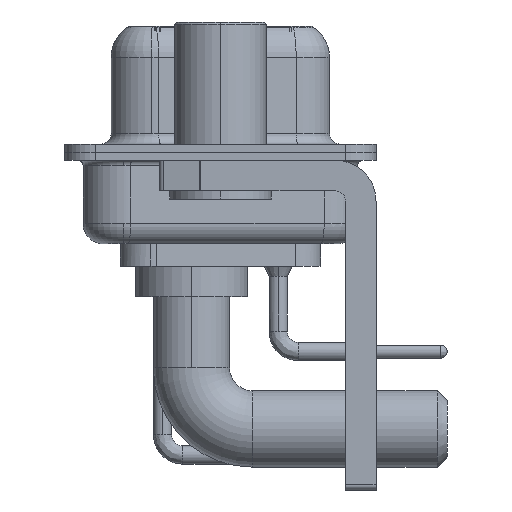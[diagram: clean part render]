
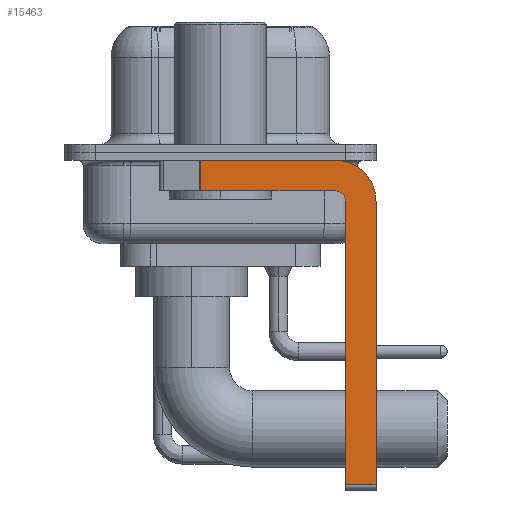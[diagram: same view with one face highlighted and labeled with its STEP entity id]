
A CAD part, left-side view. The second image highlights one B-rep face of the part: STEP entity #15463.
In plain terms, the highlighted planar face has unit normal (-1, 0, 0).
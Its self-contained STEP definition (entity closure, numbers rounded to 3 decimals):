
#171 = EDGE_LOOP ( 'NONE', ( #15192, #24403, #6575, #6069, #23442, #17105, #9714, #32960 ) ) ;
#210 = EDGE_CURVE ( 'NONE', #28596, #7166, #14443, .T. ) ;
#306 = LINE ( 'NONE', #27410, #15959 ) ;
#643 = DIRECTION ( 'NONE',  ( 0., 0., -1. ) ) ;
#693 = LINE ( 'NONE', #11523, #34291 ) ;
#996 = VERTEX_POINT ( 'NONE', #18488 ) ;
#1873 = DIRECTION ( 'NONE',  ( -1., 0., 0. ) ) ;
#3030 = VERTEX_POINT ( 'NONE', #29535 ) ;
#4671 = AXIS2_PLACEMENT_3D ( 'NONE', #13766, #25094, #643 ) ;
#4718 = DIRECTION ( 'NONE',  ( 0., 1., 0. ) ) ;
#5029 = FACE_OUTER_BOUND ( 'NONE', #171, .T. ) ;
#5260 = CARTESIAN_POINT ( 'NONE',  ( -2.9, -5.65, -0.4 ) ) ;
#6069 = ORIENTED_EDGE ( 'NONE', *, *, #210, .F. ) ;
#6180 = CARTESIAN_POINT ( 'NONE',  ( -2.9, -6.15, -2.4 ) ) ;
#6575 = ORIENTED_EDGE ( 'NONE', *, *, #10135, .F. ) ;
#7166 = VERTEX_POINT ( 'NONE', #22757 ) ;
#7369 = DIRECTION ( 'NONE',  ( 0., 0., 1. ) ) ;
#7536 = LINE ( 'NONE', #23009, #27417 ) ;
#7686 = DIRECTION ( 'NONE',  ( 1., 0., 0. ) ) ;
#7767 = DIRECTION ( 'NONE',  ( 0., 0., -1. ) ) ;
#9714 = ORIENTED_EDGE ( 'NONE', *, *, #31459, .F. ) ;
#10135 = EDGE_CURVE ( 'NONE', #7166, #24752, #7536, .T. ) ;
#10430 = LINE ( 'NONE', #24219, #21128 ) ;
#11071 = AXIS2_PLACEMENT_3D ( 'NONE', #28153, #1873, #7369 ) ;
#11468 = DIRECTION ( 'NONE',  ( 0., 0., 1. ) ) ;
#11519 = EDGE_CURVE ( 'NONE', #3030, #34802, #26026, .T. ) ;
#11523 = CARTESIAN_POINT ( 'NONE',  ( -2.9, -7.65, -2.4 ) ) ;
#11666 = EDGE_CURVE ( 'NONE', #3030, #24752, #10430, .T. ) ;
#12202 = CARTESIAN_POINT ( 'NONE',  ( -2.9, -7.65, -2.4 ) ) ;
#13766 = CARTESIAN_POINT ( 'NONE',  ( -2.9, -5.65, -2.4 ) ) ;
#14443 = CIRCLE ( 'NONE', #11071, 0.5 ) ;
#15192 = ORIENTED_EDGE ( 'NONE', *, *, #11519, .F. ) ;
#15463 = ADVANCED_FACE ( 'NONE', ( #5029 ), #23791, .F. ) ;
#15959 = VECTOR ( 'NONE', #11468, 1000. ) ;
#15987 = CIRCLE ( 'NONE', #4671, 2. ) ;
#17105 = ORIENTED_EDGE ( 'NONE', *, *, #18798, .T. ) ;
#18139 = VERTEX_POINT ( 'NONE', #12202 ) ;
#18488 = CARTESIAN_POINT ( 'NONE',  ( -2.9, -7.65, -16.35 ) ) ;
#18646 = DIRECTION ( 'NONE',  ( 0., 0., -1. ) ) ;
#18798 = EDGE_CURVE ( 'NONE', #23063, #996, #31302, .T. ) ;
#19714 = CARTESIAN_POINT ( 'NONE',  ( -2.9, 0.978, -1.9 ) ) ;
#19980 = VECTOR ( 'NONE', #20544, 1000. ) ;
#20544 = DIRECTION ( 'NONE',  ( 0., -1., 0. ) ) ;
#20997 = CARTESIAN_POINT ( 'NONE',  ( -2.9, -5.65, -16.35 ) ) ;
#21128 = VECTOR ( 'NONE', #7767, 1000. ) ;
#21418 = EDGE_CURVE ( 'NONE', #34802, #18139, #15987, .T. ) ;
#21452 = EDGE_CURVE ( 'NONE', #23063, #28596, #306, .T. ) ;
#22757 = CARTESIAN_POINT ( 'NONE',  ( -2.9, -5.65, -1.9 ) ) ;
#23009 = CARTESIAN_POINT ( 'NONE',  ( -2.9, -5.65, -1.9 ) ) ;
#23063 = VERTEX_POINT ( 'NONE', #29956 ) ;
#23442 = ORIENTED_EDGE ( 'NONE', *, *, #21452, .F. ) ;
#23791 = PLANE ( 'NONE',  #33261 ) ;
#24219 = CARTESIAN_POINT ( 'NONE',  ( -2.9, 0.978, -1.9 ) ) ;
#24403 = ORIENTED_EDGE ( 'NONE', *, *, #11666, .T. ) ;
#24752 = VERTEX_POINT ( 'NONE', #19714 ) ;
#25094 = DIRECTION ( 'NONE',  ( 1., 0., 0. ) ) ;
#25322 = DIRECTION ( 'NONE',  ( 0., 0., -1. ) ) ;
#26026 = LINE ( 'NONE', #28503, #19980 ) ;
#27139 = VECTOR ( 'NONE', #29144, 1000. ) ;
#27410 = CARTESIAN_POINT ( 'NONE',  ( -2.9, -6.15, -16.6 ) ) ;
#27417 = VECTOR ( 'NONE', #4718, 1000. ) ;
#28153 = CARTESIAN_POINT ( 'NONE',  ( -2.9, -5.65, -2.4 ) ) ;
#28503 = CARTESIAN_POINT ( 'NONE',  ( -2.9, 3., -0.4 ) ) ;
#28596 = VERTEX_POINT ( 'NONE', #6180 ) ;
#29144 = DIRECTION ( 'NONE',  ( 0., -1., 0. ) ) ;
#29535 = CARTESIAN_POINT ( 'NONE',  ( -2.9, 0.978, -0.4 ) ) ;
#29956 = CARTESIAN_POINT ( 'NONE',  ( -2.9, -6.15, -16.35 ) ) ;
#31302 = LINE ( 'NONE', #20997, #27139 ) ;
#31459 = EDGE_CURVE ( 'NONE', #18139, #996, #693, .T. ) ;
#32960 = ORIENTED_EDGE ( 'NONE', *, *, #21418, .F. ) ;
#33261 = AXIS2_PLACEMENT_3D ( 'NONE', #34635, #7686, #18646 ) ;
#34291 = VECTOR ( 'NONE', #25322, 1000. ) ;
#34635 = CARTESIAN_POINT ( 'NONE',  ( -2.9, -5.65, -2.4 ) ) ;
#34802 = VERTEX_POINT ( 'NONE', #5260 ) ;
